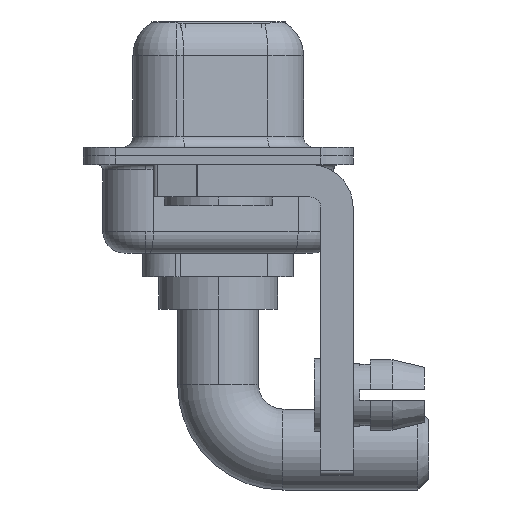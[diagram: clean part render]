
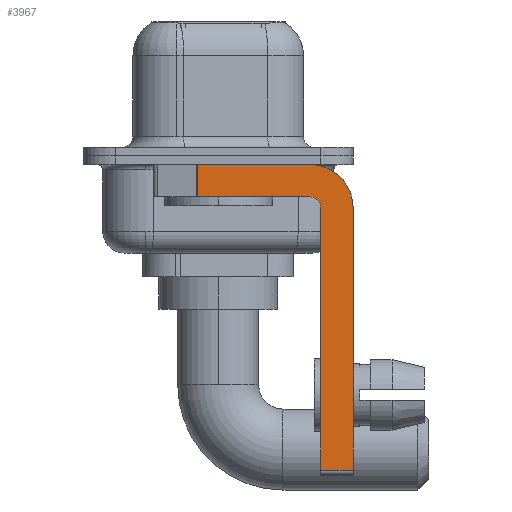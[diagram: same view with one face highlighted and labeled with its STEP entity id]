
A CAD part, left-side view. The second image highlights one B-rep face of the part: STEP entity #3967.
In plain terms, the highlighted planar face has unit normal (-1, 0, 0).
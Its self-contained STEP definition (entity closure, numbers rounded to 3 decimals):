
#379 = AXIS2_PLACEMENT_3D ( 'NONE', #8023, #6840, #12849 ) ;
#405 = VERTEX_POINT ( 'NONE', #1499 ) ;
#655 = FACE_OUTER_BOUND ( 'NONE', #4863, .T. ) ;
#959 = LINE ( 'NONE', #11811, #3695 ) ;
#1049 = CIRCLE ( 'NONE', #14464, 0.5 ) ;
#1499 = CARTESIAN_POINT ( 'NONE',  ( -2.9, -4.25, -0.4 ) ) ;
#1994 = DIRECTION ( 'NONE',  ( 0., 0., -1. ) ) ;
#2147 = CARTESIAN_POINT ( 'NONE',  ( -2.9, -4.75, -14.55 ) ) ;
#2304 = CARTESIAN_POINT ( 'NONE',  ( -2.9, -6.25, -2.4 ) ) ;
#2412 = ORIENTED_EDGE ( 'NONE', *, *, #4429, .F. ) ;
#2633 = DIRECTION ( 'NONE',  ( -1., 0., 0. ) ) ;
#2695 = CARTESIAN_POINT ( 'NONE',  ( -2.9, -4.75, -2.4 ) ) ;
#2715 = VECTOR ( 'NONE', #2859, 1000. ) ;
#2859 = DIRECTION ( 'NONE',  ( 0., 0., 1. ) ) ;
#3099 = VECTOR ( 'NONE', #6542, 1000. ) ;
#3633 = LINE ( 'NONE', #8471, #12082 ) ;
#3695 = VECTOR ( 'NONE', #10645, 1000. ) ;
#3967 = ADVANCED_FACE ( 'NONE', ( #655 ), #5500, .F. ) ;
#4018 = EDGE_CURVE ( 'NONE', #10922, #6614, #12247, .T. ) ;
#4153 = CARTESIAN_POINT ( 'NONE',  ( -2.9, -4.25, -1.9 ) ) ;
#4341 = VERTEX_POINT ( 'NONE', #13557 ) ;
#4429 = EDGE_CURVE ( 'NONE', #10922, #9620, #13715, .T. ) ;
#4636 = CARTESIAN_POINT ( 'NONE',  ( -2.9, 0.978, -0.4 ) ) ;
#4838 = CARTESIAN_POINT ( 'NONE',  ( -2.9, 0.978, -1.9 ) ) ;
#4863 = EDGE_LOOP ( 'NONE', ( #7526, #12216, #13935, #6825, #2412, #13128, #10652, #10818 ) ) ;
#5165 = CARTESIAN_POINT ( 'NONE',  ( -2.9, -4.75, -14.8 ) ) ;
#5500 = PLANE ( 'NONE',  #379 ) ;
#5564 = VERTEX_POINT ( 'NONE', #4636 ) ;
#6133 = CARTESIAN_POINT ( 'NONE',  ( -2.9, -4.25, -2.4 ) ) ;
#6277 = CARTESIAN_POINT ( 'NONE',  ( -2.9, -4.25, -2.4 ) ) ;
#6542 = DIRECTION ( 'NONE',  ( 0., -1., 0. ) ) ;
#6614 = VERTEX_POINT ( 'NONE', #9216 ) ;
#6825 = ORIENTED_EDGE ( 'NONE', *, *, #8972, .F. ) ;
#6840 = DIRECTION ( 'NONE',  ( 1., 0., 0. ) ) ;
#6866 = VERTEX_POINT ( 'NONE', #4838 ) ;
#7526 = ORIENTED_EDGE ( 'NONE', *, *, #12452, .F. ) ;
#7606 = CARTESIAN_POINT ( 'NONE',  ( -2.9, -4.25, -1.9 ) ) ;
#8023 = CARTESIAN_POINT ( 'NONE',  ( -2.9, -4.25, -2.4 ) ) ;
#8471 = CARTESIAN_POINT ( 'NONE',  ( -2.9, 3., -0.4 ) ) ;
#8634 = EDGE_CURVE ( 'NONE', #12168, #6866, #10040, .T. ) ;
#8729 = DIRECTION ( 'NONE',  ( 0., 0., -1. ) ) ;
#8972 = EDGE_CURVE ( 'NONE', #9620, #12168, #1049, .T. ) ;
#9216 = CARTESIAN_POINT ( 'NONE',  ( -2.9, -6.25, -14.55 ) ) ;
#9620 = VERTEX_POINT ( 'NONE', #2695 ) ;
#10040 = LINE ( 'NONE', #4153, #15216 ) ;
#10273 = DIRECTION ( 'NONE',  ( 0., 1., 0. ) ) ;
#10645 = DIRECTION ( 'NONE',  ( 0., 0., -1. ) ) ;
#10652 = ORIENTED_EDGE ( 'NONE', *, *, #15556, .F. ) ;
#10818 = ORIENTED_EDGE ( 'NONE', *, *, #11178, .F. ) ;
#10922 = VERTEX_POINT ( 'NONE', #2147 ) ;
#10972 = DIRECTION ( 'NONE',  ( 0., 0., 1. ) ) ;
#11159 = AXIS2_PLACEMENT_3D ( 'NONE', #6277, #13717, #8729 ) ;
#11178 = EDGE_CURVE ( 'NONE', #405, #4341, #12929, .T. ) ;
#11360 = CARTESIAN_POINT ( 'NONE',  ( -2.9, -4.25, -14.55 ) ) ;
#11811 = CARTESIAN_POINT ( 'NONE',  ( -2.9, 0.978, -1.9 ) ) ;
#11925 = EDGE_CURVE ( 'NONE', #5564, #6866, #959, .T. ) ;
#12082 = VECTOR ( 'NONE', #12267, 1000. ) ;
#12168 = VERTEX_POINT ( 'NONE', #7606 ) ;
#12216 = ORIENTED_EDGE ( 'NONE', *, *, #11925, .T. ) ;
#12247 = LINE ( 'NONE', #11360, #3099 ) ;
#12267 = DIRECTION ( 'NONE',  ( 0., -1., 0. ) ) ;
#12443 = VECTOR ( 'NONE', #1994, 1000. ) ;
#12452 = EDGE_CURVE ( 'NONE', #5564, #405, #3633, .T. ) ;
#12843 = LINE ( 'NONE', #2304, #12443 ) ;
#12849 = DIRECTION ( 'NONE',  ( 0., 0., -1. ) ) ;
#12929 = CIRCLE ( 'NONE', #11159, 2. ) ;
#13128 = ORIENTED_EDGE ( 'NONE', *, *, #4018, .T. ) ;
#13557 = CARTESIAN_POINT ( 'NONE',  ( -2.9, -6.25, -2.4 ) ) ;
#13715 = LINE ( 'NONE', #5165, #2715 ) ;
#13717 = DIRECTION ( 'NONE',  ( 1., 0., 0. ) ) ;
#13935 = ORIENTED_EDGE ( 'NONE', *, *, #8634, .F. ) ;
#14464 = AXIS2_PLACEMENT_3D ( 'NONE', #6133, #2633, #10972 ) ;
#15216 = VECTOR ( 'NONE', #10273, 1000. ) ;
#15556 = EDGE_CURVE ( 'NONE', #4341, #6614, #12843, .T. ) ;
